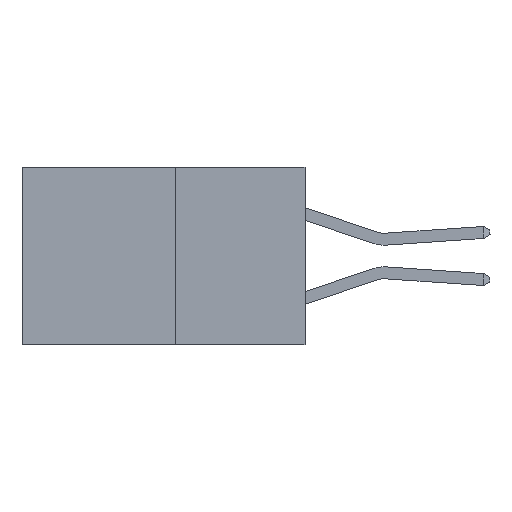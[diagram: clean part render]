
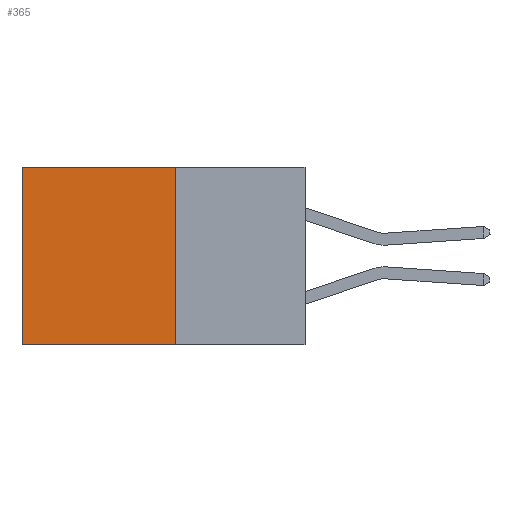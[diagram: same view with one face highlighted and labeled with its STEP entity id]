
A CAD part, left-side view. The second image highlights one B-rep face of the part: STEP entity #365.
In plain terms, the highlighted planar face has unit normal (-1, 0, 0).
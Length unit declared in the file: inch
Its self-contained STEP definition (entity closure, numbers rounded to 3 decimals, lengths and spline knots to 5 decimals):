
#127 = DIRECTION ( 'NONE',  ( 0., 0., -1. ) ) ;
#243 = VERTEX_POINT ( 'NONE', #5273 ) ;
#365 = ADVANCED_FACE ( 'NONE', ( #8181 ), #6020, .F. ) ;
#373 = ORIENTED_EDGE ( 'NONE', *, *, #7397, .T. ) ;
#954 = VECTOR ( 'NONE', #7460, 39.37008 ) ;
#1257 = DIRECTION ( 'NONE',  ( 0., 0., -1. ) ) ;
#1566 = LINE ( 'NONE', #9471, #9256 ) ;
#1677 = VERTEX_POINT ( 'NONE', #2752 ) ;
#1952 = EDGE_CURVE ( 'NONE', #5991, #243, #5265, .T. ) ;
#2179 = EDGE_LOOP ( 'NONE', ( #9292, #8624, #3828, #373 ) ) ;
#2184 = CARTESIAN_POINT ( 'NONE',  ( 0.277, 0.27, 0. ) ) ;
#2643 = EDGE_CURVE ( 'NONE', #1677, #7500, #1566, .T. ) ;
#2752 = CARTESIAN_POINT ( 'NONE',  ( 0.277, 0.59, 0. ) ) ;
#2927 = LINE ( 'NONE', #2184, #954 ) ;
#3017 = VECTOR ( 'NONE', #8546, 39.37008 ) ;
#3251 = CARTESIAN_POINT ( 'NONE',  ( 0.277, 0.27, -0.37 ) ) ;
#3828 = ORIENTED_EDGE ( 'NONE', *, *, #1952, .F. ) ;
#3867 = CARTESIAN_POINT ( 'NONE',  ( 0.277, 0.27, 0. ) ) ;
#4042 = CARTESIAN_POINT ( 'NONE',  ( 0.277, 0.27, -0.37 ) ) ;
#5265 = LINE ( 'NONE', #3251, #8589 ) ;
#5273 = CARTESIAN_POINT ( 'NONE',  ( 0.277, 0.27, -0.37 ) ) ;
#5669 = DIRECTION ( 'NONE',  ( 0., 0., -1. ) ) ;
#5991 = VERTEX_POINT ( 'NONE', #3867 ) ;
#6020 = PLANE ( 'NONE',  #7549 ) ;
#6198 = DIRECTION ( 'NONE',  ( 1., 0., 0. ) ) ;
#6785 = CARTESIAN_POINT ( 'NONE',  ( 0.277, 0.59, -0.37 ) ) ;
#6957 = CARTESIAN_POINT ( 'NONE',  ( 0.277, 0.27, -0.37 ) ) ;
#7397 = EDGE_CURVE ( 'NONE', #5991, #1677, #2927, .T. ) ;
#7460 = DIRECTION ( 'NONE',  ( 0., 1., 0. ) ) ;
#7500 = VERTEX_POINT ( 'NONE', #6785 ) ;
#7549 = AXIS2_PLACEMENT_3D ( 'NONE', #6957, #6198, #5669 ) ;
#8181 = FACE_OUTER_BOUND ( 'NONE', #2179, .T. ) ;
#8546 = DIRECTION ( 'NONE',  ( 0., 1., 0. ) ) ;
#8589 = VECTOR ( 'NONE', #1257, 39.37008 ) ;
#8624 = ORIENTED_EDGE ( 'NONE', *, *, #9631, .F. ) ;
#8958 = LINE ( 'NONE', #4042, #3017 ) ;
#9256 = VECTOR ( 'NONE', #127, 39.37008 ) ;
#9292 = ORIENTED_EDGE ( 'NONE', *, *, #2643, .T. ) ;
#9471 = CARTESIAN_POINT ( 'NONE',  ( 0.277, 0.59, -0.37 ) ) ;
#9631 = EDGE_CURVE ( 'NONE', #243, #7500, #8958, .T. ) ;
